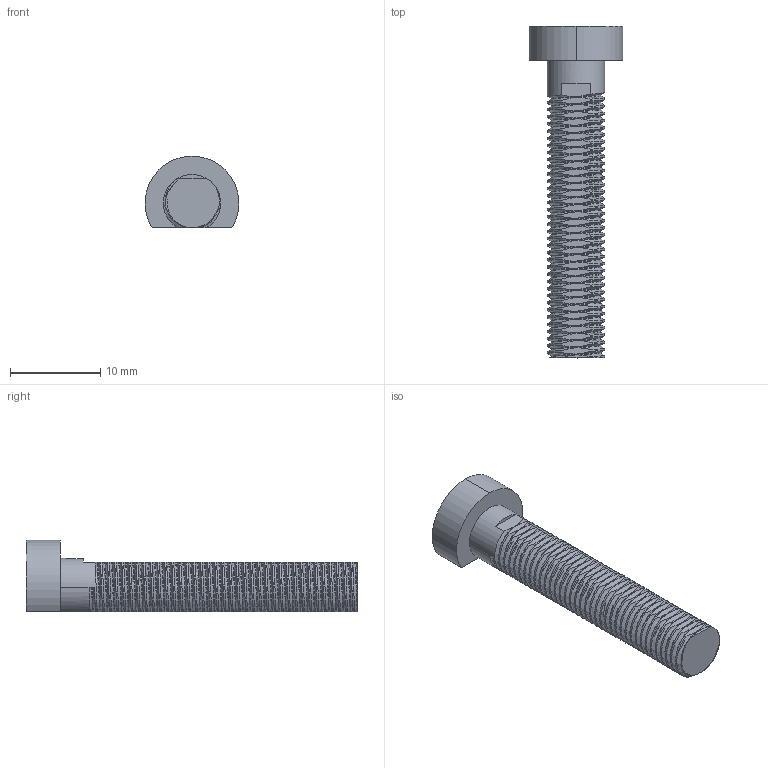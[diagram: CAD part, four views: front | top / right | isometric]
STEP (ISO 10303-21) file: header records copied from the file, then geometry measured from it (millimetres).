
FILE_DESCRIPTION (( 'STEP AP203' ), '1' );
FILE_NAME ('AF-WF-GS-PRT-009-STEP.STEP', '2020-07-21T20:13:53', ( '' ), ( '' ), 'SwSTEP 2.0', 'SolidWorks 2018', '' );
FILE_SCHEMA (( 'CONFIG_CONTROL_DESIGN' ));
Length unit declared in the file: inch
Products named in the file (1): AF-WF-GS-PRT-009-STEP
Bounding box: 10.39 x 36.83 x 7.95 mm (x, y, z)
Volume: 1156.9 mm3; surface area: 1180.9 mm2
Topology: 1 solids, 1 shells, 206 faces, 607 edges, 404 vertices
Faces by surface type: cylinder 119, plane 84, bspline 3
Entity records: 13126 total; most frequent: CARTESIAN_POINT 8531, ORIENTED_EDGE 1214, DIRECTION 652, EDGE_CURVE 607, VERTEX_POINT 404, AXIS2_PLACEMENT_3D 220, LINE 212, VECTOR 212
